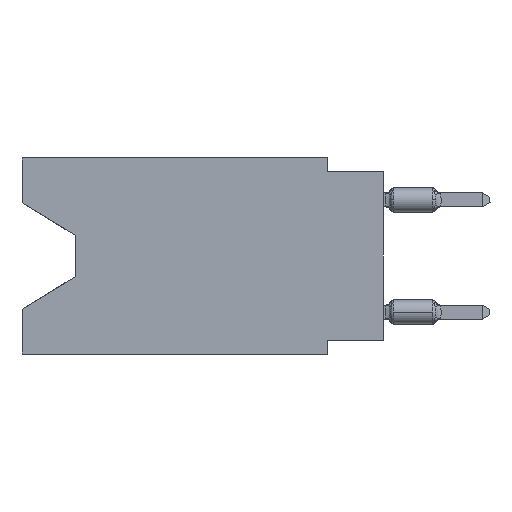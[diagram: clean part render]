
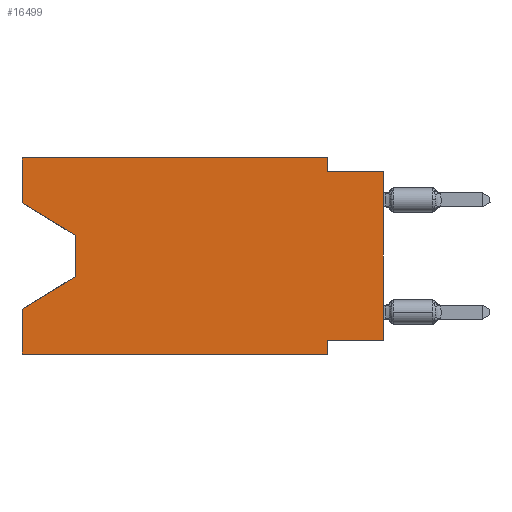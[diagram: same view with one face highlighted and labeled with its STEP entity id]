
A CAD part, left-side view. The second image highlights one B-rep face of the part: STEP entity #16499.
In plain terms, the highlighted planar face has unit normal (-1, 0, 0).
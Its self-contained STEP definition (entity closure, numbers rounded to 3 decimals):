
#150 = CARTESIAN_POINT ( 'NONE',  ( 0., 2.54, -8.89 ) ) ;
#189 = DIRECTION ( 'NONE',  ( 0., 0., 1. ) ) ;
#231 = VERTEX_POINT ( 'NONE', #11957 ) ;
#296 = CARTESIAN_POINT ( 'NONE',  ( 0., 16.383, 0. ) ) ;
#573 = VECTOR ( 'NONE', #3016, 1000. ) ;
#606 = DIRECTION ( 'NONE',  ( 0., 0., -1. ) ) ;
#900 = CARTESIAN_POINT ( 'NONE',  ( 0., 13.97, -3.505 ) ) ;
#1286 = DIRECTION ( 'NONE',  ( 0., 0.855, -0.519 ) ) ;
#1371 = DIRECTION ( 'NONE',  ( 0., 0., -1. ) ) ;
#1494 = ORIENTED_EDGE ( 'NONE', *, *, #5349, .F. ) ;
#1725 = EDGE_CURVE ( 'NONE', #10865, #6513, #11037, .T. ) ;
#2086 = VECTOR ( 'NONE', #3753, 1000. ) ;
#2187 = AXIS2_PLACEMENT_3D ( 'NONE', #15770, #8390, #1371 ) ;
#2526 = CARTESIAN_POINT ( 'NONE',  ( 0., 2.54, -8.255 ) ) ;
#2530 = CARTESIAN_POINT ( 'NONE',  ( 0., 13.97, -5.385 ) ) ;
#2566 = VECTOR ( 'NONE', #21670, 1000. ) ;
#2679 = CARTESIAN_POINT ( 'NONE',  ( 0., 0., -0.635 ) ) ;
#3016 = DIRECTION ( 'NONE',  ( 0., -1., 0. ) ) ;
#3487 = ORIENTED_EDGE ( 'NONE', *, *, #22910, .F. ) ;
#3693 = EDGE_CURVE ( 'NONE', #4572, #14501, #17436, .T. ) ;
#3753 = DIRECTION ( 'NONE',  ( 0., 0., 1. ) ) ;
#3881 = EDGE_CURVE ( 'NONE', #19621, #10865, #11221, .T. ) ;
#3970 = VERTEX_POINT ( 'NONE', #8054 ) ;
#4135 = DIRECTION ( 'NONE',  ( 0., -1., 0. ) ) ;
#4572 = VERTEX_POINT ( 'NONE', #2530 ) ;
#4894 = CARTESIAN_POINT ( 'NONE',  ( 0., 16.383, -6.852 ) ) ;
#5346 = VERTEX_POINT ( 'NONE', #15552 ) ;
#5349 = EDGE_CURVE ( 'NONE', #12026, #14309, #8064, .T. ) ;
#5377 = CARTESIAN_POINT ( 'NONE',  ( 0., 0., -8.255 ) ) ;
#6513 = VERTEX_POINT ( 'NONE', #15810 ) ;
#6899 = CARTESIAN_POINT ( 'NONE',  ( 0., 13.97, -5.385 ) ) ;
#6966 = EDGE_CURVE ( 'NONE', #20797, #8275, #21471, .T. ) ;
#7082 = DIRECTION ( 'NONE',  ( 0., -0.855, -0.519 ) ) ;
#7378 = CARTESIAN_POINT ( 'NONE',  ( 0., 16.383, 0. ) ) ;
#7841 = EDGE_LOOP ( 'NONE', ( #16332, #19929, #21365, #17792, #16371, #17285, #16212, #9055, #1494, #14311, #12615, #3487 ) ) ;
#7901 = VECTOR ( 'NONE', #16948, 1000. ) ;
#8054 = CARTESIAN_POINT ( 'NONE',  ( 0., 16.383, 0. ) ) ;
#8064 = LINE ( 'NONE', #2679, #7901 ) ;
#8275 = VERTEX_POINT ( 'NONE', #900 ) ;
#8336 = LINE ( 'NONE', #13842, #15735 ) ;
#8390 = DIRECTION ( 'NONE',  ( 1., 0., 0. ) ) ;
#9005 = CARTESIAN_POINT ( 'NONE',  ( 0., 13.97, -3.505 ) ) ;
#9055 = ORIENTED_EDGE ( 'NONE', *, *, #18663, .T. ) ;
#9103 = EDGE_CURVE ( 'NONE', #8275, #4572, #10646, .T. ) ;
#9205 = LINE ( 'NONE', #296, #11204 ) ;
#9506 = LINE ( 'NONE', #13135, #10649 ) ;
#9915 = FACE_OUTER_BOUND ( 'NONE', #7841, .T. ) ;
#10265 = PLANE ( 'NONE',  #2187 ) ;
#10646 = LINE ( 'NONE', #9005, #13803 ) ;
#10649 = VECTOR ( 'NONE', #606, 1000. ) ;
#10675 = EDGE_CURVE ( 'NONE', #231, #6513, #20788, .T. ) ;
#10865 = VERTEX_POINT ( 'NONE', #2526 ) ;
#11037 = LINE ( 'NONE', #150, #2566 ) ;
#11204 = VECTOR ( 'NONE', #189, 1000. ) ;
#11221 = LINE ( 'NONE', #5377, #16454 ) ;
#11957 = CARTESIAN_POINT ( 'NONE',  ( 0., 16.383, -8.89 ) ) ;
#12026 = VERTEX_POINT ( 'NONE', #13633 ) ;
#12615 = ORIENTED_EDGE ( 'NONE', *, *, #22646, .F. ) ;
#12817 = CARTESIAN_POINT ( 'NONE',  ( 0., 16.383, -2.038 ) ) ;
#13135 = CARTESIAN_POINT ( 'NONE',  ( 0., 2.54, 0. ) ) ;
#13460 = VECTOR ( 'NONE', #1286, 1000. ) ;
#13633 = CARTESIAN_POINT ( 'NONE',  ( 0., 2.54, -0.635 ) ) ;
#13803 = VECTOR ( 'NONE', #19533, 1000. ) ;
#13831 = EDGE_CURVE ( 'NONE', #5346, #12026, #9506, .T. ) ;
#13842 = CARTESIAN_POINT ( 'NONE',  ( 0., 0., 0. ) ) ;
#14309 = VERTEX_POINT ( 'NONE', #18361 ) ;
#14311 = ORIENTED_EDGE ( 'NONE', *, *, #13831, .F. ) ;
#14501 = VERTEX_POINT ( 'NONE', #4894 ) ;
#15552 = CARTESIAN_POINT ( 'NONE',  ( 0., 2.54, 0. ) ) ;
#15735 = VECTOR ( 'NONE', #21189, 1000. ) ;
#15770 = CARTESIAN_POINT ( 'NONE',  ( 0., 16.383, 0. ) ) ;
#15810 = CARTESIAN_POINT ( 'NONE',  ( 0., 2.54, -8.89 ) ) ;
#16087 = CARTESIAN_POINT ( 'NONE',  ( 0., 0., -8.255 ) ) ;
#16212 = ORIENTED_EDGE ( 'NONE', *, *, #3881, .F. ) ;
#16332 = ORIENTED_EDGE ( 'NONE', *, *, #6966, .T. ) ;
#16371 = ORIENTED_EDGE ( 'NONE', *, *, #10675, .T. ) ;
#16454 = VECTOR ( 'NONE', #19990, 1000. ) ;
#16499 = ADVANCED_FACE ( 'NONE', ( #9915 ), #10265, .F. ) ;
#16948 = DIRECTION ( 'NONE',  ( 0., -1., 0. ) ) ;
#17098 = CARTESIAN_POINT ( 'NONE',  ( 0., 16.383, 0. ) ) ;
#17285 = ORIENTED_EDGE ( 'NONE', *, *, #1725, .F. ) ;
#17436 = LINE ( 'NONE', #6899, #13460 ) ;
#17792 = ORIENTED_EDGE ( 'NONE', *, *, #17910, .F. ) ;
#17910 = EDGE_CURVE ( 'NONE', #231, #14501, #9205, .T. ) ;
#18361 = CARTESIAN_POINT ( 'NONE',  ( 0., 0., -0.635 ) ) ;
#18518 = LINE ( 'NONE', #17098, #21124 ) ;
#18663 = EDGE_CURVE ( 'NONE', #19621, #14309, #8336, .T. ) ;
#19036 = CARTESIAN_POINT ( 'NONE',  ( 0., 16.383, -8.89 ) ) ;
#19260 = CARTESIAN_POINT ( 'NONE',  ( 0., 16.383, -2.038 ) ) ;
#19533 = DIRECTION ( 'NONE',  ( 0., 0., -1. ) ) ;
#19621 = VERTEX_POINT ( 'NONE', #16087 ) ;
#19929 = ORIENTED_EDGE ( 'NONE', *, *, #9103, .T. ) ;
#19990 = DIRECTION ( 'NONE',  ( 0., 1., 0. ) ) ;
#20788 = LINE ( 'NONE', #19036, #573 ) ;
#20797 = VERTEX_POINT ( 'NONE', #12817 ) ;
#21124 = VECTOR ( 'NONE', #4135, 1000. ) ;
#21189 = DIRECTION ( 'NONE',  ( 0., 0., 1. ) ) ;
#21302 = VECTOR ( 'NONE', #7082, 1000. ) ;
#21365 = ORIENTED_EDGE ( 'NONE', *, *, #3693, .T. ) ;
#21471 = LINE ( 'NONE', #19260, #21302 ) ;
#21645 = LINE ( 'NONE', #7378, #2086 ) ;
#21670 = DIRECTION ( 'NONE',  ( 0., 0., -1. ) ) ;
#22646 = EDGE_CURVE ( 'NONE', #3970, #5346, #18518, .T. ) ;
#22910 = EDGE_CURVE ( 'NONE', #20797, #3970, #21645, .T. ) ;
